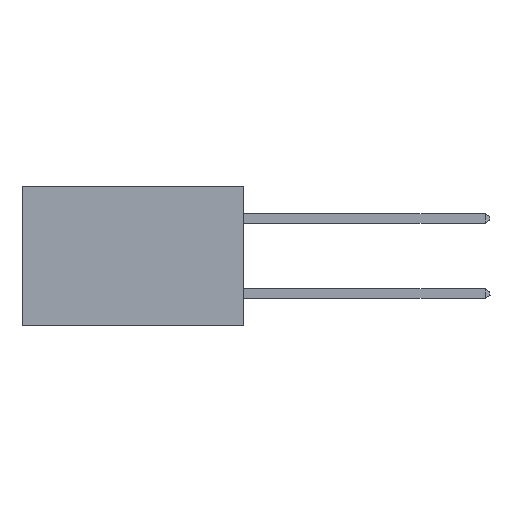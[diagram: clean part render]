
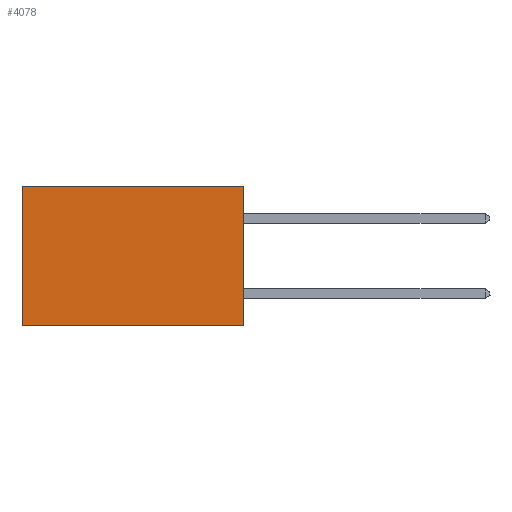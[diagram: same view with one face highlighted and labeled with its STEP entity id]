
A CAD part, left-side view. The second image highlights one B-rep face of the part: STEP entity #4078.
In plain terms, the highlighted planar face has unit normal (-1, 0, 0).
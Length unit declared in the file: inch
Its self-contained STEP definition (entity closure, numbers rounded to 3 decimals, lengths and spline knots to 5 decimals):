
#109 = LINE ( 'NONE', #7998, #10980 ) ;
#1073 = VECTOR ( 'NONE', #12039, 39.37008 ) ;
#2491 = AXIS2_PLACEMENT_3D ( 'NONE', #16636, #16819, #16734 ) ;
#4078 = ADVANCED_FACE ( 'NONE', ( #21771 ), #16884, .F. ) ;
#4492 = EDGE_CURVE ( 'NONE', #22736, #23843, #5283, .T. ) ;
#4501 = ORIENTED_EDGE ( 'NONE', *, *, #23484, .T. ) ;
#5283 = LINE ( 'NONE', #20999, #21745 ) ;
#5562 = ORIENTED_EDGE ( 'NONE', *, *, #13782, .T. ) ;
#6611 = CARTESIAN_POINT ( 'NONE',  ( 0.277, 0., 0. ) ) ;
#7770 = CARTESIAN_POINT ( 'NONE',  ( 0.277, 0.59, -0.37 ) ) ;
#7998 = CARTESIAN_POINT ( 'NONE',  ( 0.277, 0., 0. ) ) ;
#8819 = DIRECTION ( 'NONE',  ( 0., 1., 0. ) ) ;
#9307 = VECTOR ( 'NONE', #8819, 39.37008 ) ;
#9883 = VERTEX_POINT ( 'NONE', #20874 ) ;
#10980 = VECTOR ( 'NONE', #14469, 39.37008 ) ;
#12039 = DIRECTION ( 'NONE',  ( 0., 0., -1. ) ) ;
#12577 = LINE ( 'NONE', #7770, #1073 ) ;
#12897 = EDGE_LOOP ( 'NONE', ( #5562, #21476, #16887, #4501 ) ) ;
#13341 = CARTESIAN_POINT ( 'NONE',  ( 0.277, 0., -0.37 ) ) ;
#13782 = EDGE_CURVE ( 'NONE', #18242, #9883, #12577, .T. ) ;
#14469 = DIRECTION ( 'NONE',  ( 0., 1., 0. ) ) ;
#16636 = CARTESIAN_POINT ( 'NONE',  ( 0.277, 0., -0.37 ) ) ;
#16734 = DIRECTION ( 'NONE',  ( 0., 0., -1. ) ) ;
#16819 = DIRECTION ( 'NONE',  ( 1., 0., 0. ) ) ;
#16884 = PLANE ( 'NONE',  #2491 ) ;
#16887 = ORIENTED_EDGE ( 'NONE', *, *, #4492, .F. ) ;
#18242 = VERTEX_POINT ( 'NONE', #23132 ) ;
#19995 = LINE ( 'NONE', #21629, #9307 ) ;
#20656 = DIRECTION ( 'NONE',  ( 0., 0., -1. ) ) ;
#20874 = CARTESIAN_POINT ( 'NONE',  ( 0.277, 0.59, -0.37 ) ) ;
#20999 = CARTESIAN_POINT ( 'NONE',  ( 0.277, 0., -0.37 ) ) ;
#21476 = ORIENTED_EDGE ( 'NONE', *, *, #26866, .F. ) ;
#21629 = CARTESIAN_POINT ( 'NONE',  ( 0.277, 0., -0.37 ) ) ;
#21745 = VECTOR ( 'NONE', #20656, 39.37008 ) ;
#21771 = FACE_OUTER_BOUND ( 'NONE', #12897, .T. ) ;
#22736 = VERTEX_POINT ( 'NONE', #6611 ) ;
#23132 = CARTESIAN_POINT ( 'NONE',  ( 0.277, 0.59, 0. ) ) ;
#23484 = EDGE_CURVE ( 'NONE', #22736, #18242, #109, .T. ) ;
#23843 = VERTEX_POINT ( 'NONE', #13341 ) ;
#26866 = EDGE_CURVE ( 'NONE', #23843, #9883, #19995, .T. ) ;
